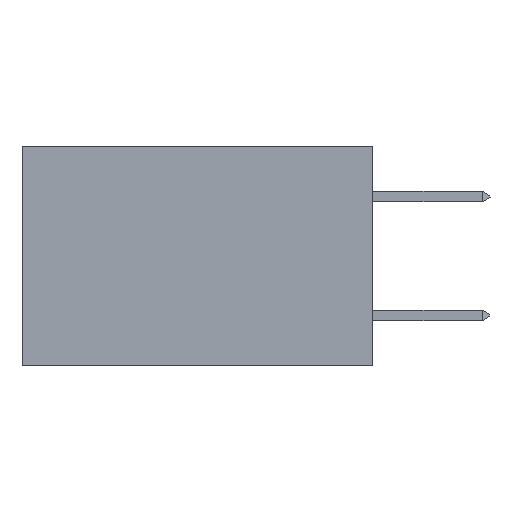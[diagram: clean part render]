
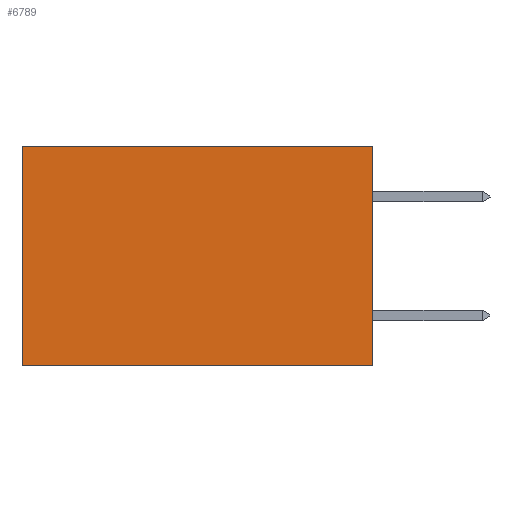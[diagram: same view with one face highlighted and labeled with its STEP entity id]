
A CAD part, left-side view. The second image highlights one B-rep face of the part: STEP entity #6789.
In plain terms, the highlighted planar face has unit normal (-1, 0, 0).
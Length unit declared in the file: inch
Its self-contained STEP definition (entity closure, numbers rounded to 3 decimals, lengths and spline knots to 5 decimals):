
#440 = DIRECTION ( 'NONE',  ( 1., 0., 0. ) ) ;
#657 = EDGE_CURVE ( 'NONE', #7685, #8998, #8698, .T. ) ;
#786 = CARTESIAN_POINT ( 'NONE',  ( 0.277, 0.59, 0. ) ) ;
#822 = ORIENTED_EDGE ( 'NONE', *, *, #7163, .F. ) ;
#843 = ORIENTED_EDGE ( 'NONE', *, *, #5892, .T. ) ;
#849 = CARTESIAN_POINT ( 'NONE',  ( 0.277, 0.59, -0.37 ) ) ;
#931 = CARTESIAN_POINT ( 'NONE',  ( 0.277, 0., 0. ) ) ;
#1036 = DIRECTION ( 'NONE',  ( 0., 1., 0. ) ) ;
#1252 = EDGE_LOOP ( 'NONE', ( #843, #822, #4298, #3138 ) ) ;
#1552 = LINE ( 'NONE', #3663, #7087 ) ;
#1647 = CARTESIAN_POINT ( 'NONE',  ( 0.277, 0., -0.37 ) ) ;
#1664 = VERTEX_POINT ( 'NONE', #8197 ) ;
#2520 = EDGE_CURVE ( 'NONE', #7685, #6548, #1552, .T. ) ;
#2690 = AXIS2_PLACEMENT_3D ( 'NONE', #4808, #440, #5498 ) ;
#2831 = VECTOR ( 'NONE', #5391, 39.37008 ) ;
#2836 = DIRECTION ( 'NONE',  ( 0., 0., -1. ) ) ;
#2940 = FACE_OUTER_BOUND ( 'NONE', #1252, .T. ) ;
#3138 = ORIENTED_EDGE ( 'NONE', *, *, #2520, .T. ) ;
#3236 = DIRECTION ( 'NONE',  ( 0., 1., 0. ) ) ;
#3381 = VECTOR ( 'NONE', #3236, 39.37008 ) ;
#3663 = CARTESIAN_POINT ( 'NONE',  ( 0.277, 0., 0. ) ) ;
#4298 = ORIENTED_EDGE ( 'NONE', *, *, #657, .F. ) ;
#4808 = CARTESIAN_POINT ( 'NONE',  ( 0.277, 0., -0.37 ) ) ;
#4811 = CARTESIAN_POINT ( 'NONE',  ( 0.277, 0., -0.37 ) ) ;
#5391 = DIRECTION ( 'NONE',  ( 0., 0., -1. ) ) ;
#5498 = DIRECTION ( 'NONE',  ( 0., 0., -1. ) ) ;
#5892 = EDGE_CURVE ( 'NONE', #6548, #1664, #8065, .T. ) ;
#6053 = CARTESIAN_POINT ( 'NONE',  ( 0.277, 0., -0.37 ) ) ;
#6548 = VERTEX_POINT ( 'NONE', #786 ) ;
#6789 = ADVANCED_FACE ( 'NONE', ( #2940 ), #9009, .F. ) ;
#7087 = VECTOR ( 'NONE', #1036, 39.37008 ) ;
#7163 = EDGE_CURVE ( 'NONE', #8998, #1664, #8976, .T. ) ;
#7685 = VERTEX_POINT ( 'NONE', #931 ) ;
#7864 = VECTOR ( 'NONE', #2836, 39.37008 ) ;
#8065 = LINE ( 'NONE', #849, #7864 ) ;
#8197 = CARTESIAN_POINT ( 'NONE',  ( 0.277, 0.59, -0.37 ) ) ;
#8698 = LINE ( 'NONE', #1647, #2831 ) ;
#8976 = LINE ( 'NONE', #6053, #3381 ) ;
#8998 = VERTEX_POINT ( 'NONE', #4811 ) ;
#9009 = PLANE ( 'NONE',  #2690 ) ;
